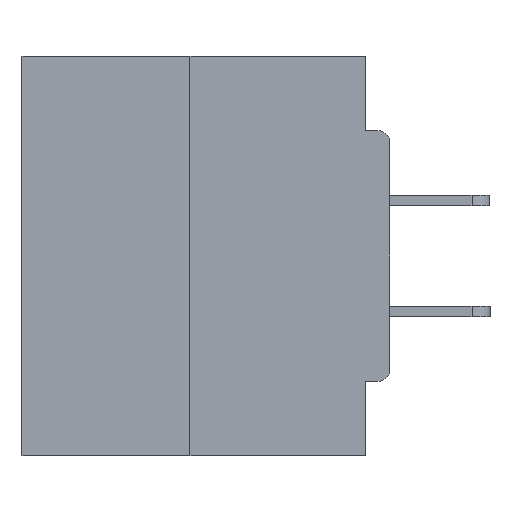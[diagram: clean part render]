
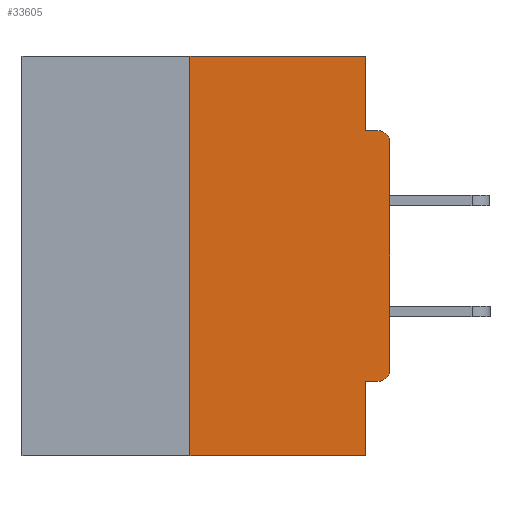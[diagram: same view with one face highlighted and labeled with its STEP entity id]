
A CAD part, left-side view. The second image highlights one B-rep face of the part: STEP entity #33605.
In plain terms, the highlighted planar face has unit normal (-1, 0, 0).
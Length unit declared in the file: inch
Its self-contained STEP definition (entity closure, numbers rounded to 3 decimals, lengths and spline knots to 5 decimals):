
#334 = DIRECTION ( 'NONE',  ( 0., 0., 1. ) ) ;
#864 = CARTESIAN_POINT ( 'NONE',  ( 0., 0.25, -0.5 ) ) ;
#985 = DIRECTION ( 'NONE',  ( 0., 0., -1. ) ) ;
#1539 = VERTEX_POINT ( 'NONE', #33153 ) ;
#1651 = EDGE_CURVE ( 'NONE', #33070, #13431, #12149, .T. ) ;
#1918 = VECTOR ( 'NONE', #5572, 39.37008 ) ;
#2425 = CARTESIAN_POINT ( 'NONE',  ( 0., 0.015, -0.1085 ) ) ;
#3026 = ORIENTED_EDGE ( 'NONE', *, *, #18551, .F. ) ;
#3076 = CARTESIAN_POINT ( 'NONE',  ( 0., 0.031, -0.5 ) ) ;
#3366 = ORIENTED_EDGE ( 'NONE', *, *, #18544, .F. ) ;
#3511 = VECTOR ( 'NONE', #4795, 39.37008 ) ;
#3893 = VERTEX_POINT ( 'NONE', #4214 ) ;
#3947 = DIRECTION ( 'NONE',  ( 0., -1., 0. ) ) ;
#4214 = CARTESIAN_POINT ( 'NONE',  ( 0., 0.031, -0.5 ) ) ;
#4656 = AXIS2_PLACEMENT_3D ( 'NONE', #21681, #8118, #8356 ) ;
#4795 = DIRECTION ( 'NONE',  ( 0., 0., 1. ) ) ;
#5572 = DIRECTION ( 'NONE',  ( 0., -1., 0. ) ) ;
#6246 = VECTOR ( 'NONE', #32878, 39.37008 ) ;
#6357 = CARTESIAN_POINT ( 'NONE',  ( 0., 0., -0.0935 ) ) ;
#6891 = LINE ( 'NONE', #28903, #3511 ) ;
#6943 = ORIENTED_EDGE ( 'NONE', *, *, #29104, .T. ) ;
#6999 = VERTEX_POINT ( 'NONE', #864 ) ;
#7046 = CARTESIAN_POINT ( 'NONE',  ( 0., 0.015, -0.0935 ) ) ;
#7948 = LINE ( 'NONE', #3076, #6246 ) ;
#8012 = CARTESIAN_POINT ( 'NONE',  ( 0., 0.25, 0. ) ) ;
#8074 = CARTESIAN_POINT ( 'NONE',  ( 0., 0.46, -0.5 ) ) ;
#8118 = DIRECTION ( 'NONE',  ( 1., 0., 0. ) ) ;
#8154 = VECTOR ( 'NONE', #3947, 39.37008 ) ;
#8356 = DIRECTION ( 'NONE',  ( 0., 0., -1. ) ) ;
#9017 = CARTESIAN_POINT ( 'NONE',  ( 0., 0.015, -0.3915 ) ) ;
#9306 = AXIS2_PLACEMENT_3D ( 'NONE', #2425, #13276, #26879 ) ;
#9768 = CARTESIAN_POINT ( 'NONE',  ( 0., 0., -0.4065 ) ) ;
#10167 = EDGE_CURVE ( 'NONE', #33070, #20152, #15986, .T. ) ;
#10713 = LINE ( 'NONE', #25584, #23361 ) ;
#10973 = ORIENTED_EDGE ( 'NONE', *, *, #24293, .T. ) ;
#10992 = VERTEX_POINT ( 'NONE', #26985 ) ;
#11238 = CARTESIAN_POINT ( 'NONE',  ( 0., 0.031, 0. ) ) ;
#11686 = DIRECTION ( 'NONE',  ( 0., -1., 0. ) ) ;
#11706 = CARTESIAN_POINT ( 'NONE',  ( 0., 0.015, -0.4065 ) ) ;
#11739 = DIRECTION ( 'NONE',  ( -1., 0., 0. ) ) ;
#12149 = CIRCLE ( 'NONE', #27565, 0.015 ) ;
#12709 = DIRECTION ( 'NONE',  ( 0., 1., 0. ) ) ;
#13276 = DIRECTION ( 'NONE',  ( -1., 0., 0. ) ) ;
#13431 = VERTEX_POINT ( 'NONE', #27929 ) ;
#14170 = LINE ( 'NONE', #8074, #1918 ) ;
#14918 = ORIENTED_EDGE ( 'NONE', *, *, #28626, .F. ) ;
#15664 = ORIENTED_EDGE ( 'NONE', *, *, #24035, .F. ) ;
#15986 = LINE ( 'NONE', #9768, #26559 ) ;
#16275 = VERTEX_POINT ( 'NONE', #11238 ) ;
#17438 = LINE ( 'NONE', #8012, #33524 ) ;
#17880 = LINE ( 'NONE', #20007, #8154 ) ;
#18544 = EDGE_CURVE ( 'NONE', #10992, #16275, #17880, .T. ) ;
#18551 = EDGE_CURVE ( 'NONE', #16275, #1539, #10713, .T. ) ;
#19738 = EDGE_LOOP ( 'NONE', ( #3366, #14918, #30673, #20935, #22810, #34329, #10973, #6943, #15664, #3026 ) ) ;
#20007 = CARTESIAN_POINT ( 'NONE',  ( 0., 0.46, 0. ) ) ;
#20152 = VERTEX_POINT ( 'NONE', #29039 ) ;
#20239 = DIRECTION ( 'NONE',  ( 0., 0., -1. ) ) ;
#20935 = ORIENTED_EDGE ( 'NONE', *, *, #29785, .F. ) ;
#21569 = PLANE ( 'NONE',  #4656 ) ;
#21681 = CARTESIAN_POINT ( 'NONE',  ( 0., 0.46, 0. ) ) ;
#22810 = ORIENTED_EDGE ( 'NONE', *, *, #10167, .F. ) ;
#23361 = VECTOR ( 'NONE', #20239, 39.37008 ) ;
#24035 = EDGE_CURVE ( 'NONE', #1539, #27940, #27190, .T. ) ;
#24293 = EDGE_CURVE ( 'NONE', #13431, #26750, #6891, .T. ) ;
#25584 = CARTESIAN_POINT ( 'NONE',  ( 0., 0.031, 0. ) ) ;
#26559 = VECTOR ( 'NONE', #12709, 39.37008 ) ;
#26750 = VERTEX_POINT ( 'NONE', #28978 ) ;
#26797 = VECTOR ( 'NONE', #11686, 39.37008 ) ;
#26879 = DIRECTION ( 'NONE',  ( 0., 0., -1. ) ) ;
#26985 = CARTESIAN_POINT ( 'NONE',  ( 0., 0.25, 0. ) ) ;
#27190 = LINE ( 'NONE', #6357, #26797 ) ;
#27565 = AXIS2_PLACEMENT_3D ( 'NONE', #9017, #11739, #985 ) ;
#27929 = CARTESIAN_POINT ( 'NONE',  ( 0., 0., -0.3915 ) ) ;
#27940 = VERTEX_POINT ( 'NONE', #7046 ) ;
#28626 = EDGE_CURVE ( 'NONE', #6999, #10992, #17438, .T. ) ;
#28903 = CARTESIAN_POINT ( 'NONE',  ( 0., 0., 0. ) ) ;
#28978 = CARTESIAN_POINT ( 'NONE',  ( 0., 0., -0.1085 ) ) ;
#29039 = CARTESIAN_POINT ( 'NONE',  ( 0., 0.031, -0.4065 ) ) ;
#29104 = EDGE_CURVE ( 'NONE', #26750, #27940, #30350, .T. ) ;
#29785 = EDGE_CURVE ( 'NONE', #20152, #3893, #7948, .T. ) ;
#30350 = CIRCLE ( 'NONE', #9306, 0.015 ) ;
#30673 = ORIENTED_EDGE ( 'NONE', *, *, #31032, .T. ) ;
#31032 = EDGE_CURVE ( 'NONE', #6999, #3893, #14170, .T. ) ;
#32878 = DIRECTION ( 'NONE',  ( 0., 0., -1. ) ) ;
#33070 = VERTEX_POINT ( 'NONE', #11706 ) ;
#33153 = CARTESIAN_POINT ( 'NONE',  ( 0., 0.031, -0.0935 ) ) ;
#33331 = FACE_OUTER_BOUND ( 'NONE', #19738, .T. ) ;
#33524 = VECTOR ( 'NONE', #334, 39.37008 ) ;
#33605 = ADVANCED_FACE ( 'NONE', ( #33331 ), #21569, .F. ) ;
#34329 = ORIENTED_EDGE ( 'NONE', *, *, #1651, .T. ) ;
